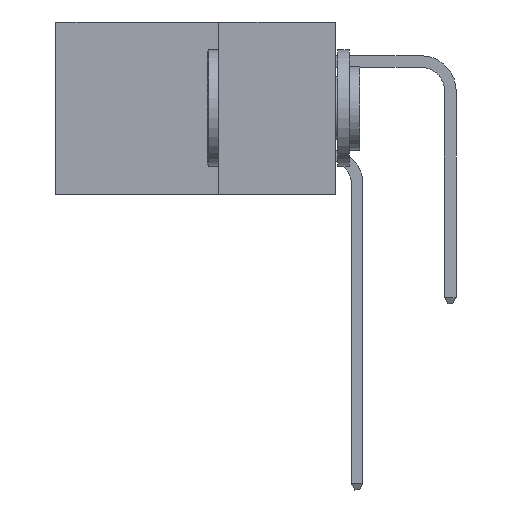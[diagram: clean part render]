
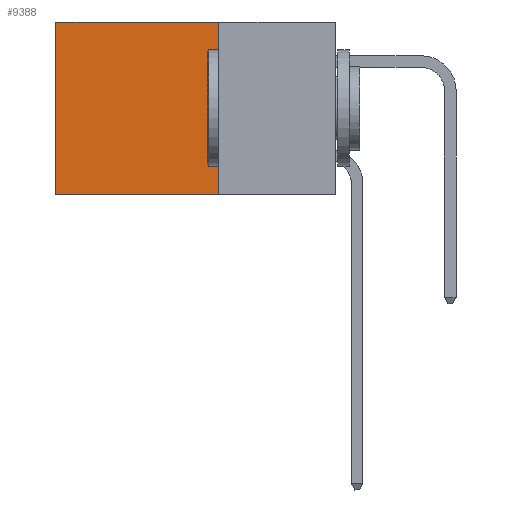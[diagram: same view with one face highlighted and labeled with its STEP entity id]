
A CAD part, left-side view. The second image highlights one B-rep face of the part: STEP entity #9388.
In plain terms, the highlighted planar face has unit normal (-1, 0, 0).
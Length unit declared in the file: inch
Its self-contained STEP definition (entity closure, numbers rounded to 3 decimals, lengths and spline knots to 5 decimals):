
#882 = ORIENTED_EDGE ( 'NONE', *, *, #17479, .T. ) ;
#1110 = DIRECTION ( 'NONE',  ( 0., 0., -1. ) ) ;
#1243 = EDGE_CURVE ( 'NONE', #11073, #4388, #14054, .T. ) ;
#1346 = DIRECTION ( 'NONE',  ( 1., 0., 0. ) ) ;
#2289 = CARTESIAN_POINT ( 'NONE',  ( 0.2875, 0.6, 0. ) ) ;
#4388 = VERTEX_POINT ( 'NONE', #14706 ) ;
#4914 = VECTOR ( 'NONE', #17321, 39.37008 ) ;
#5786 = LINE ( 'NONE', #9184, #16321 ) ;
#6342 = DIRECTION ( 'NONE',  ( 0., 0., -1. ) ) ;
#6618 = LINE ( 'NONE', #10917, #4914 ) ;
#7127 = LINE ( 'NONE', #16571, #19642 ) ;
#8961 = AXIS2_PLACEMENT_3D ( 'NONE', #15380, #1346, #12284 ) ;
#9184 = CARTESIAN_POINT ( 'NONE',  ( 0.2875, 0.25, 0. ) ) ;
#9239 = CARTESIAN_POINT ( 'NONE',  ( 0.2875, 0.25, 0. ) ) ;
#9388 = ADVANCED_FACE ( 'NONE', ( #18673 ), #13943, .F. ) ;
#9801 = ORIENTED_EDGE ( 'NONE', *, *, #1243, .F. ) ;
#10917 = CARTESIAN_POINT ( 'NONE',  ( 0.2875, 0.25, -0.37 ) ) ;
#10977 = EDGE_LOOP ( 'NONE', ( #882, #19506, #9801, #13313 ) ) ;
#11073 = VERTEX_POINT ( 'NONE', #19786 ) ;
#12284 = DIRECTION ( 'NONE',  ( 0., 0., -1. ) ) ;
#12834 = VERTEX_POINT ( 'NONE', #19952 ) ;
#13087 = EDGE_CURVE ( 'NONE', #4388, #12834, #6618, .T. ) ;
#13313 = ORIENTED_EDGE ( 'NONE', *, *, #15263, .T. ) ;
#13917 = VERTEX_POINT ( 'NONE', #2289 ) ;
#13943 = PLANE ( 'NONE',  #8961 ) ;
#14054 = LINE ( 'NONE', #9239, #18956 ) ;
#14706 = CARTESIAN_POINT ( 'NONE',  ( 0.2875, 0.25, -0.37 ) ) ;
#15263 = EDGE_CURVE ( 'NONE', #11073, #13917, #5786, .T. ) ;
#15380 = CARTESIAN_POINT ( 'NONE',  ( 0.2875, 0.25, 0. ) ) ;
#16321 = VECTOR ( 'NONE', #20127, 39.37008 ) ;
#16571 = CARTESIAN_POINT ( 'NONE',  ( 0.2875, 0.6, 0. ) ) ;
#17321 = DIRECTION ( 'NONE',  ( 0., 1., 0. ) ) ;
#17479 = EDGE_CURVE ( 'NONE', #13917, #12834, #7127, .T. ) ;
#18673 = FACE_OUTER_BOUND ( 'NONE', #10977, .T. ) ;
#18956 = VECTOR ( 'NONE', #6342, 39.37008 ) ;
#19506 = ORIENTED_EDGE ( 'NONE', *, *, #13087, .F. ) ;
#19642 = VECTOR ( 'NONE', #1110, 39.37008 ) ;
#19786 = CARTESIAN_POINT ( 'NONE',  ( 0.2875, 0.25, 0. ) ) ;
#19952 = CARTESIAN_POINT ( 'NONE',  ( 0.2875, 0.6, -0.37 ) ) ;
#20127 = DIRECTION ( 'NONE',  ( 0., 1., 0. ) ) ;
